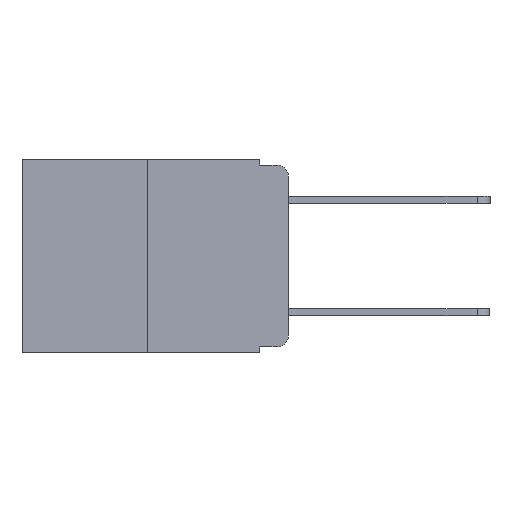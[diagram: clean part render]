
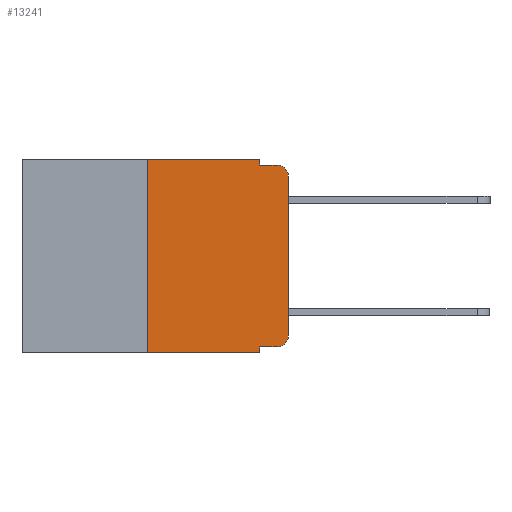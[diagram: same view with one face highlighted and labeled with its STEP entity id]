
A CAD part, left-side view. The second image highlights one B-rep face of the part: STEP entity #13241.
In plain terms, the highlighted planar face has unit normal (-1, 0, 0).
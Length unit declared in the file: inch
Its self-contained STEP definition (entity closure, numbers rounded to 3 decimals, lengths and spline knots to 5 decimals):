
#345 = EDGE_CURVE ( 'NONE', #2225, #763, #13082, .T. ) ;
#406 = ORIENTED_EDGE ( 'NONE', *, *, #5892, .T. ) ;
#642 = ORIENTED_EDGE ( 'NONE', *, *, #5972, .F. ) ;
#763 = VERTEX_POINT ( 'NONE', #11501 ) ;
#1331 = LINE ( 'NONE', #4223, #12395 ) ;
#1433 = CARTESIAN_POINT ( 'NONE',  ( 0., 0., -0.03 ) ) ;
#1520 = VERTEX_POINT ( 'NONE', #6649 ) ;
#1708 = VECTOR ( 'NONE', #6409, 39.37008 ) ;
#1788 = ORIENTED_EDGE ( 'NONE', *, *, #6659, .T. ) ;
#1800 = CARTESIAN_POINT ( 'NONE',  ( 0., 0., 0. ) ) ;
#1883 = LINE ( 'NONE', #12038, #10280 ) ;
#1960 = CARTESIAN_POINT ( 'NONE',  ( 0., 0.02, -0.313 ) ) ;
#2069 = EDGE_CURVE ( 'NONE', #6948, #3610, #3440, .T. ) ;
#2204 = CARTESIAN_POINT ( 'NONE',  ( 0., 0.473, 0. ) ) ;
#2210 = CARTESIAN_POINT ( 'NONE',  ( 0., 0.25, 0. ) ) ;
#2225 = VERTEX_POINT ( 'NONE', #4202 ) ;
#2519 = CARTESIAN_POINT ( 'NONE',  ( 0., 0.051, -0.01 ) ) ;
#2643 = CARTESIAN_POINT ( 'NONE',  ( 0., 0.02, -0.03 ) ) ;
#3128 = DIRECTION ( 'NONE',  ( 0., 0., -1. ) ) ;
#3231 = VERTEX_POINT ( 'NONE', #3575 ) ;
#3440 = LINE ( 'NONE', #7546, #8967 ) ;
#3575 = CARTESIAN_POINT ( 'NONE',  ( 0., 0.051, -0.343 ) ) ;
#3610 = VERTEX_POINT ( 'NONE', #2210 ) ;
#3847 = DIRECTION ( 'NONE',  ( 0., 0., -1. ) ) ;
#3853 = PLANE ( 'NONE',  #13664 ) ;
#4202 = CARTESIAN_POINT ( 'NONE',  ( 0., 0.051, 0. ) ) ;
#4223 = CARTESIAN_POINT ( 'NONE',  ( 0., 0.473, -0.343 ) ) ;
#4412 = VERTEX_POINT ( 'NONE', #1433 ) ;
#4427 = EDGE_CURVE ( 'NONE', #10261, #3231, #5186, .T. ) ;
#4449 = CIRCLE ( 'NONE', #5980, 0.02 ) ;
#4465 = AXIS2_PLACEMENT_3D ( 'NONE', #2643, #10258, #3847 ) ;
#4556 = CARTESIAN_POINT ( 'NONE',  ( 0., 0.051, 0. ) ) ;
#4875 = EDGE_CURVE ( 'NONE', #6948, #3231, #1331, .T. ) ;
#4970 = DIRECTION ( 'NONE',  ( 0., 0., -1. ) ) ;
#5186 = LINE ( 'NONE', #4556, #10480 ) ;
#5538 = CARTESIAN_POINT ( 'NONE',  ( 0., 0.051, 0. ) ) ;
#5542 = DIRECTION ( 'NONE',  ( 0., -1., 0. ) ) ;
#5783 = VERTEX_POINT ( 'NONE', #13059 ) ;
#5892 = EDGE_CURVE ( 'NONE', #10261, #1520, #1883, .T. ) ;
#5972 = EDGE_CURVE ( 'NONE', #763, #5783, #6532, .T. ) ;
#5980 = AXIS2_PLACEMENT_3D ( 'NONE', #1960, #9680, #3128 ) ;
#6040 = DIRECTION ( 'NONE',  ( 0., -1., 0. ) ) ;
#6409 = DIRECTION ( 'NONE',  ( 0., 0., 1. ) ) ;
#6532 = LINE ( 'NONE', #2519, #11631 ) ;
#6649 = CARTESIAN_POINT ( 'NONE',  ( 0., 0.02, -0.333 ) ) ;
#6659 = EDGE_CURVE ( 'NONE', #1520, #13262, #4449, .T. ) ;
#6948 = VERTEX_POINT ( 'NONE', #12918 ) ;
#7029 = DIRECTION ( 'NONE',  ( 0., 0., -1. ) ) ;
#7277 = ORIENTED_EDGE ( 'NONE', *, *, #12187, .T. ) ;
#7476 = DIRECTION ( 'NONE',  ( 0., 0., 1. ) ) ;
#7546 = CARTESIAN_POINT ( 'NONE',  ( 0., 0.25, 0. ) ) ;
#7699 = ORIENTED_EDGE ( 'NONE', *, *, #8337, .F. ) ;
#7862 = FACE_OUTER_BOUND ( 'NONE', #12714, .T. ) ;
#7940 = ORIENTED_EDGE ( 'NONE', *, *, #2069, .F. ) ;
#8211 = CARTESIAN_POINT ( 'NONE',  ( 0., 0.473, 0. ) ) ;
#8337 = EDGE_CURVE ( 'NONE', #3610, #2225, #12010, .T. ) ;
#8426 = ORIENTED_EDGE ( 'NONE', *, *, #345, .F. ) ;
#8620 = ORIENTED_EDGE ( 'NONE', *, *, #4427, .F. ) ;
#8967 = VECTOR ( 'NONE', #7476, 39.37008 ) ;
#9680 = DIRECTION ( 'NONE',  ( -1., 0., 0. ) ) ;
#9758 = DIRECTION ( 'NONE',  ( 0., 0., -1. ) ) ;
#10258 = DIRECTION ( 'NONE',  ( -1., 0., 0. ) ) ;
#10261 = VERTEX_POINT ( 'NONE', #11828 ) ;
#10280 = VECTOR ( 'NONE', #11837, 39.37008 ) ;
#10441 = LINE ( 'NONE', #1800, #1708 ) ;
#10480 = VECTOR ( 'NONE', #7029, 39.37008 ) ;
#11223 = DIRECTION ( 'NONE',  ( 1., 0., 0. ) ) ;
#11341 = EDGE_CURVE ( 'NONE', #4412, #5783, #12232, .T. ) ;
#11501 = CARTESIAN_POINT ( 'NONE',  ( 0., 0.051, -0.01 ) ) ;
#11631 = VECTOR ( 'NONE', #11647, 39.37008 ) ;
#11647 = DIRECTION ( 'NONE',  ( 0., -1., 0. ) ) ;
#11721 = VECTOR ( 'NONE', #5542, 39.37008 ) ;
#11828 = CARTESIAN_POINT ( 'NONE',  ( 0., 0.051, -0.333 ) ) ;
#11837 = DIRECTION ( 'NONE',  ( 0., -1., 0. ) ) ;
#12010 = LINE ( 'NONE', #2204, #11721 ) ;
#12038 = CARTESIAN_POINT ( 'NONE',  ( 0., 0.051, -0.333 ) ) ;
#12162 = CARTESIAN_POINT ( 'NONE',  ( 0., 0., -0.313 ) ) ;
#12187 = EDGE_CURVE ( 'NONE', #13262, #4412, #10441, .T. ) ;
#12232 = CIRCLE ( 'NONE', #4465, 0.02 ) ;
#12395 = VECTOR ( 'NONE', #6040, 39.37008 ) ;
#12439 = ORIENTED_EDGE ( 'NONE', *, *, #11341, .T. ) ;
#12714 = EDGE_LOOP ( 'NONE', ( #7277, #12439, #642, #8426, #7699, #7940, #13172, #8620, #406, #1788 ) ) ;
#12918 = CARTESIAN_POINT ( 'NONE',  ( 0., 0.25, -0.343 ) ) ;
#13059 = CARTESIAN_POINT ( 'NONE',  ( 0., 0.02, -0.01 ) ) ;
#13082 = LINE ( 'NONE', #5538, #13370 ) ;
#13172 = ORIENTED_EDGE ( 'NONE', *, *, #4875, .T. ) ;
#13241 = ADVANCED_FACE ( 'NONE', ( #7862 ), #3853, .F. ) ;
#13262 = VERTEX_POINT ( 'NONE', #12162 ) ;
#13370 = VECTOR ( 'NONE', #9758, 39.37008 ) ;
#13664 = AXIS2_PLACEMENT_3D ( 'NONE', #8211, #11223, #4970 ) ;
